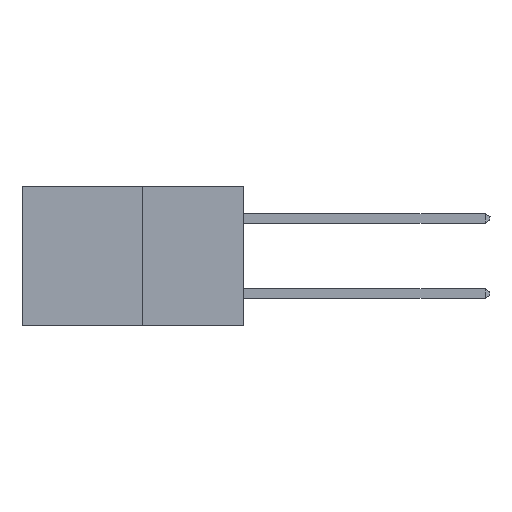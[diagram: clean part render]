
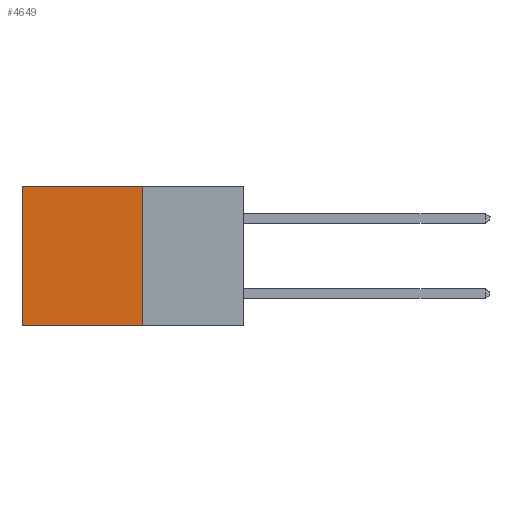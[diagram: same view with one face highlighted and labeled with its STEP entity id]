
A CAD part, left-side view. The second image highlights one B-rep face of the part: STEP entity #4649.
In plain terms, the highlighted planar face has unit normal (-1, 0, 0).
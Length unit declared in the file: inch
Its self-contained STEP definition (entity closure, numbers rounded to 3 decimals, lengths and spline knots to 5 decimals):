
#79 = DIRECTION ( 'NONE',  ( 1., 0., 0. ) ) ;
#359 = CARTESIAN_POINT ( 'NONE',  ( 0.277, 0.27, -0.37 ) ) ;
#1074 = VERTEX_POINT ( 'NONE', #2214 ) ;
#1081 = CARTESIAN_POINT ( 'NONE',  ( 0.277, 0.59, 0. ) ) ;
#1410 = VECTOR ( 'NONE', #4857, 39.37008 ) ;
#1497 = EDGE_CURVE ( 'NONE', #1703, #4633, #1697, .T. ) ;
#1697 = LINE ( 'NONE', #4841, #1410 ) ;
#1703 = VERTEX_POINT ( 'NONE', #1081 ) ;
#1794 = EDGE_CURVE ( 'NONE', #1074, #3064, #7357, .T. ) ;
#1914 = ORIENTED_EDGE ( 'NONE', *, *, #9743, .T. ) ;
#2032 = ORIENTED_EDGE ( 'NONE', *, *, #8711, .F. ) ;
#2214 = CARTESIAN_POINT ( 'NONE',  ( 0.277, 0.27, 0. ) ) ;
#2906 = DIRECTION ( 'NONE',  ( 0., 1., 0. ) ) ;
#3006 = ORIENTED_EDGE ( 'NONE', *, *, #1497, .T. ) ;
#3064 = VERTEX_POINT ( 'NONE', #4565 ) ;
#3353 = CARTESIAN_POINT ( 'NONE',  ( 0.277, 0.59, -0.37 ) ) ;
#4208 = LINE ( 'NONE', #5099, #5760 ) ;
#4283 = ORIENTED_EDGE ( 'NONE', *, *, #1794, .F. ) ;
#4565 = CARTESIAN_POINT ( 'NONE',  ( 0.277, 0.27, -0.37 ) ) ;
#4633 = VERTEX_POINT ( 'NONE', #3353 ) ;
#4649 = ADVANCED_FACE ( 'NONE', ( #8228 ), #4847, .F. ) ;
#4713 = AXIS2_PLACEMENT_3D ( 'NONE', #8678, #79, #5702 ) ;
#4841 = CARTESIAN_POINT ( 'NONE',  ( 0.277, 0.59, -0.37 ) ) ;
#4847 = PLANE ( 'NONE',  #4713 ) ;
#4857 = DIRECTION ( 'NONE',  ( 0., 0., -1. ) ) ;
#5099 = CARTESIAN_POINT ( 'NONE',  ( 0.277, 0.27, -0.37 ) ) ;
#5462 = LINE ( 'NONE', #6725, #9214 ) ;
#5702 = DIRECTION ( 'NONE',  ( 0., 0., -1. ) ) ;
#5760 = VECTOR ( 'NONE', #9563, 39.37008 ) ;
#6725 = CARTESIAN_POINT ( 'NONE',  ( 0.277, 0.27, 0. ) ) ;
#7357 = LINE ( 'NONE', #359, #7580 ) ;
#7580 = VECTOR ( 'NONE', #9909, 39.37008 ) ;
#8228 = FACE_OUTER_BOUND ( 'NONE', #9340, .T. ) ;
#8678 = CARTESIAN_POINT ( 'NONE',  ( 0.277, 0.27, -0.37 ) ) ;
#8711 = EDGE_CURVE ( 'NONE', #3064, #4633, #4208, .T. ) ;
#9214 = VECTOR ( 'NONE', #2906, 39.37008 ) ;
#9340 = EDGE_LOOP ( 'NONE', ( #3006, #2032, #4283, #1914 ) ) ;
#9563 = DIRECTION ( 'NONE',  ( 0., 1., 0. ) ) ;
#9743 = EDGE_CURVE ( 'NONE', #1074, #1703, #5462, .T. ) ;
#9909 = DIRECTION ( 'NONE',  ( 0., 0., -1. ) ) ;
